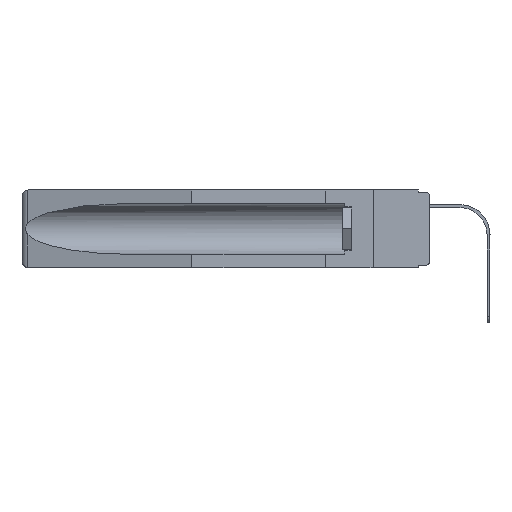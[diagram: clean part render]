
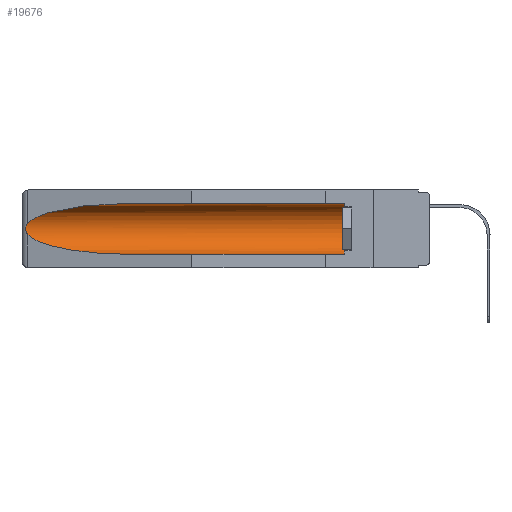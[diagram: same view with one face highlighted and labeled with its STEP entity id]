
A CAD part, left-side view. The second image highlights one B-rep face of the part: STEP entity #19676.
In plain terms, the highlighted cylindrical face has radius 2.857 mm (diameter 5.715 mm), a partial arc.
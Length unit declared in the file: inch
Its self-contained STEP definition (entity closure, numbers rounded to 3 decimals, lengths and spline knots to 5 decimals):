
#60 = CARTESIAN_POINT ( 'NONE',  ( 0.2675, 1.53308, -0.17534 ) ) ;
#370 = EDGE_CURVE ( 'NONE', #13489, #7719, #16256, .T. ) ;
#380 = AXIS2_PLACEMENT_3D ( 'NONE', #18748, #5520, #7396 ) ;
#827 = CARTESIAN_POINT ( 'NONE',  ( 0.155, -0.30754, -0.1715 ) ) ;
#895 = EDGE_LOOP ( 'NONE', ( #5130, #4133, #1747, #15446, #20573, #4071 ) ) ;
#1119 = CARTESIAN_POINT ( 'NONE',  ( 0.21114, 1.30732, -0.059 ) ) ;
#1345 = CARTESIAN_POINT ( 'NONE',  ( 0.26537, 1.52718, -0.19328 ) ) ;
#1684 = EDGE_CURVE ( 'NONE', #2095, #5973, #4745, .T. ) ;
#1747 = ORIENTED_EDGE ( 'NONE', *, *, #370, .T. ) ;
#1912 = VECTOR ( 'NONE', #11241, 39.37008 ) ;
#2095 = VERTEX_POINT ( 'NONE', #3727 ) ;
#3087 = CARTESIAN_POINT ( 'NONE',  ( 0.155, 1.07973, -0.284 ) ) ;
#3176 = DIRECTION ( 'NONE',  ( 0., 1., 0. ) ) ;
#3489 = LINE ( 'NONE', #9945, #9434 ) ;
#3683 = CARTESIAN_POINT ( 'NONE',  ( 0.155, 1.07973, -0.284 ) ) ;
#3727 = CARTESIAN_POINT ( 'NONE',  ( 0.155, 1.07973, -0.059 ) ) ;
#3955 = EDGE_CURVE ( 'NONE', #12579, #9652, #19678, .T. ) ;
#3979 = CARTESIAN_POINT ( 'NONE',  ( 0.155, 0.126, -0.059 ) ) ;
#4071 = ORIENTED_EDGE ( 'NONE', *, *, #14775, .T. ) ;
#4133 = ORIENTED_EDGE ( 'NONE', *, *, #19794, .T. ) ;
#4631 = CARTESIAN_POINT ( 'NONE',  ( 0.26537, 1.52718, -0.14972 ) ) ;
#4745 =( BOUNDED_CURVE ( )  B_SPLINE_CURVE ( 3, ( #15639, #1119, #7572, #14047 ),
 .UNSPECIFIED., .F., .T. ) 
 B_SPLINE_CURVE_WITH_KNOTS ( ( 4, 4 ),
 ( 4.71239, 6.08839 ),
 .UNSPECIFIED. ) 
 CURVE ( )  GEOMETRIC_REPRESENTATION_ITEM ( )  RATIONAL_B_SPLINE_CURVE ( ( 1., 0.848, 0.848, 1. ) ) 
 REPRESENTATION_ITEM ( '' )  );
#5130 = ORIENTED_EDGE ( 'NONE', *, *, #1684, .T. ) ;
#5520 = DIRECTION ( 'NONE',  ( 0., -1., 0. ) ) ;
#5802 = FACE_OUTER_BOUND ( 'NONE', #895, .T. ) ;
#5973 = VERTEX_POINT ( 'NONE', #18010 ) ;
#6319 = CARTESIAN_POINT ( 'NONE',  ( 0.26655, 1.53094, -0.18657 ) ) ;
#6528 = CARTESIAN_POINT ( 'NONE',  ( 0.2675, 1.53308, -0.16763 ) ) ;
#6549 = AXIS2_PLACEMENT_3D ( 'NONE', #827, #17236, #7288 ) ;
#7288 = DIRECTION ( 'NONE',  ( 0., 0., 1. ) ) ;
#7396 = DIRECTION ( 'NONE',  ( 0., 0., 1. ) ) ;
#7572 = CARTESIAN_POINT ( 'NONE',  ( 0.25451, 1.48313, -0.09465 ) ) ;
#7719 = VERTEX_POINT ( 'NONE', #3683 ) ;
#8190 = CARTESIAN_POINT ( 'NONE',  ( 0.155, 0.126, -0.284 ) ) ;
#9402 = CARTESIAN_POINT ( 'NONE',  ( 0.2673, 1.5327, -0.16383 ) ) ;
#9434 = VECTOR ( 'NONE', #3176, 39.37008 ) ;
#9652 = VERTEX_POINT ( 'NONE', #3979 ) ;
#9766 = CARTESIAN_POINT ( 'NONE',  ( 0.155, -0.30754, -0.059 ) ) ;
#9945 = CARTESIAN_POINT ( 'NONE',  ( 0.155, -0.30754, -0.284 ) ) ;
#11241 = DIRECTION ( 'NONE',  ( 0., 1., 0. ) ) ;
#12169 = EDGE_CURVE ( 'NONE', #12579, #7719, #3489, .T. ) ;
#12579 = VERTEX_POINT ( 'NONE', #8190 ) ;
#12731 = CARTESIAN_POINT ( 'NONE',  ( 0.26537, 1.52718, -0.19328 ) ) ;
#13489 = VERTEX_POINT ( 'NONE', #16019 ) ;
#14047 = CARTESIAN_POINT ( 'NONE',  ( 0.26537, 1.52718, -0.14972 ) ) ;
#14324 = CARTESIAN_POINT ( 'NONE',  ( 0.25451, 1.48313, -0.24835 ) ) ;
#14385 = CARTESIAN_POINT ( 'NONE',  ( 0.26597, 1.5296, -0.19026 ) ) ;
#14775 = EDGE_CURVE ( 'NONE', #9652, #2095, #20678, .T. ) ;
#15343 = CYLINDRICAL_SURFACE ( 'NONE', #6549, 0.1125 ) ;
#15446 = ORIENTED_EDGE ( 'NONE', *, *, #12169, .F. ) ;
#15639 = CARTESIAN_POINT ( 'NONE',  ( 0.155, 1.07973, -0.059 ) ) ;
#15865 = CARTESIAN_POINT ( 'NONE',  ( 0.26654, 1.53092, -0.15636 ) ) ;
#16017 = CARTESIAN_POINT ( 'NONE',  ( 0.21114, 1.30732, -0.284 ) ) ;
#16019 = CARTESIAN_POINT ( 'NONE',  ( 0.26537, 1.52718, -0.19328 ) ) ;
#16256 =( BOUNDED_CURVE ( )  B_SPLINE_CURVE ( 3, ( #12731, #14324, #16017, #3087 ),
 .UNSPECIFIED., .F., .T. ) 
 B_SPLINE_CURVE_WITH_KNOTS ( ( 4, 4 ),
 ( 0.1948, 1.5708 ),
 .UNSPECIFIED. ) 
 CURVE ( )  GEOMETRIC_REPRESENTATION_ITEM ( )  RATIONAL_B_SPLINE_CURVE ( ( 1., 0.848, 0.848, 1. ) ) 
 REPRESENTATION_ITEM ( '' )  );
#17236 = DIRECTION ( 'NONE',  ( 0., 1., 0. ) ) ;
#17532 = B_SPLINE_CURVE_WITH_KNOTS ( 'NONE', 3,
 ( #4631, #20726, #15865, #9402, #6528, #60, #17871, #6319, #14385, #1345 ),
 .UNSPECIFIED., .F., .F.,
 ( 4, 2, 2, 2, 4 ),
 ( 0., 0.00029, 0.00058, 0.00087, 0.00117 ),
 .UNSPECIFIED. ) ;
#17871 = CARTESIAN_POINT ( 'NONE',  ( 0.2673, 1.53269, -0.17917 ) ) ;
#18010 = CARTESIAN_POINT ( 'NONE',  ( 0.26537, 1.52718, -0.14972 ) ) ;
#18748 = CARTESIAN_POINT ( 'NONE',  ( 0.155, 0.126, -0.1715 ) ) ;
#19676 = ADVANCED_FACE ( 'NONE', ( #5802 ), #15343, .F. ) ;
#19678 = CIRCLE ( 'NONE', #380, 0.1125 ) ;
#19794 = EDGE_CURVE ( 'NONE', #5973, #13489, #17532, .T. ) ;
#20573 = ORIENTED_EDGE ( 'NONE', *, *, #3955, .T. ) ;
#20678 = LINE ( 'NONE', #9766, #1912 ) ;
#20726 = CARTESIAN_POINT ( 'NONE',  ( 0.26597, 1.52961, -0.15275 ) ) ;
